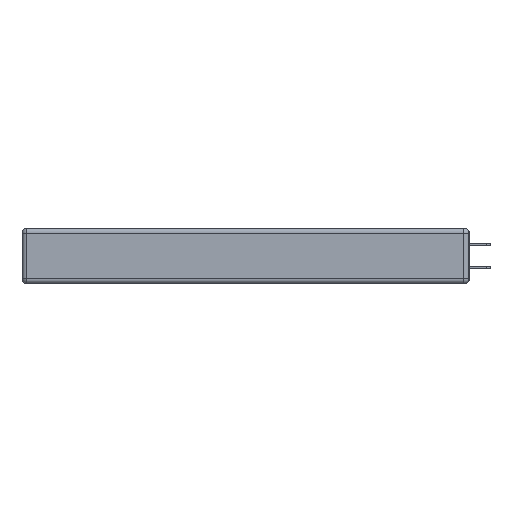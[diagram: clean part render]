
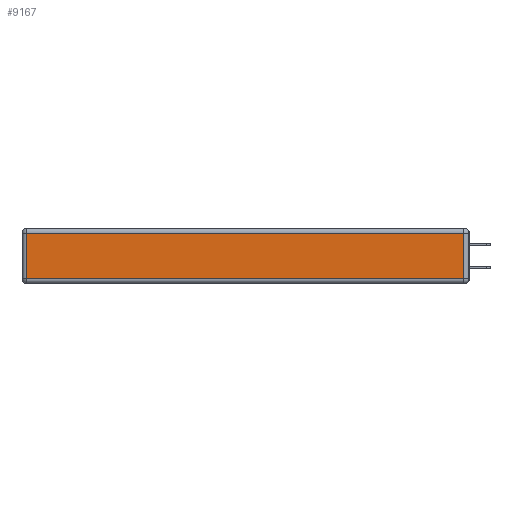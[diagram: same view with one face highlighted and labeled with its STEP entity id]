
A CAD part, left-side view. The second image highlights one B-rep face of the part: STEP entity #9167.
In plain terms, the highlighted planar face has unit normal (-1, 0, 0).
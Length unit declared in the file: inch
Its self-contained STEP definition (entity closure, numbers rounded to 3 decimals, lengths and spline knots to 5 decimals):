
#218 = PLANE ( 'NONE',  #24675 ) ;
#305 = DIRECTION ( 'NONE',  ( 0., 0., 1. ) ) ;
#1964 = VECTOR ( 'NONE', #5734, 39.37008 ) ;
#2726 = LINE ( 'NONE', #7223, #8931 ) ;
#2805 = CARTESIAN_POINT ( 'NONE',  ( 0., 0.03, -0.03 ) ) ;
#3046 = ORIENTED_EDGE ( 'NONE', *, *, #26388, .T. ) ;
#4100 = CARTESIAN_POINT ( 'NONE',  ( 0., 2.72, -0.343 ) ) ;
#4257 = LINE ( 'NONE', #4100, #1964 ) ;
#5115 = DIRECTION ( 'NONE',  ( 0., -1., 0. ) ) ;
#5734 = DIRECTION ( 'NONE',  ( 0., 0., -1. ) ) ;
#6194 = VERTEX_POINT ( 'NONE', #24801 ) ;
#7223 = CARTESIAN_POINT ( 'NONE',  ( 0., 0.03, -0.343 ) ) ;
#8496 = VECTOR ( 'NONE', #19951, 39.37008 ) ;
#8931 = VECTOR ( 'NONE', #13575, 39.37008 ) ;
#8938 = VERTEX_POINT ( 'NONE', #22077 ) ;
#9052 = CARTESIAN_POINT ( 'NONE',  ( 0., 0., -0.313 ) ) ;
#9167 = ADVANCED_FACE ( 'NONE', ( #10372 ), #218, .T. ) ;
#10372 = FACE_OUTER_BOUND ( 'NONE', #12320, .T. ) ;
#10502 = CARTESIAN_POINT ( 'NONE',  ( 0., 2.72, -0.313 ) ) ;
#11140 = VERTEX_POINT ( 'NONE', #10502 ) ;
#12320 = EDGE_LOOP ( 'NONE', ( #23861, #25351, #3046, #17737 ) ) ;
#12808 = DIRECTION ( 'NONE',  ( -1., 0., 0. ) ) ;
#13537 = VECTOR ( 'NONE', #5115, 39.37008 ) ;
#13575 = DIRECTION ( 'NONE',  ( 0., 0., 1. ) ) ;
#14387 = EDGE_CURVE ( 'NONE', #11140, #6194, #20064, .T. ) ;
#17737 = ORIENTED_EDGE ( 'NONE', *, *, #22283, .T. ) ;
#19107 = CARTESIAN_POINT ( 'NONE',  ( 0., 0., -0.343 ) ) ;
#19428 = VERTEX_POINT ( 'NONE', #2805 ) ;
#19571 = LINE ( 'NONE', #26121, #8496 ) ;
#19951 = DIRECTION ( 'NONE',  ( 0., 1., 0. ) ) ;
#20064 = LINE ( 'NONE', #9052, #13537 ) ;
#22077 = CARTESIAN_POINT ( 'NONE',  ( 0., 2.72, -0.03 ) ) ;
#22283 = EDGE_CURVE ( 'NONE', #8938, #11140, #4257, .T. ) ;
#23861 = ORIENTED_EDGE ( 'NONE', *, *, #14387, .T. ) ;
#24136 = EDGE_CURVE ( 'NONE', #6194, #19428, #2726, .T. ) ;
#24675 = AXIS2_PLACEMENT_3D ( 'NONE', #19107, #12808, #305 ) ;
#24801 = CARTESIAN_POINT ( 'NONE',  ( 0., 0.03, -0.313 ) ) ;
#25351 = ORIENTED_EDGE ( 'NONE', *, *, #24136, .T. ) ;
#26121 = CARTESIAN_POINT ( 'NONE',  ( 0., 2.75, -0.03 ) ) ;
#26388 = EDGE_CURVE ( 'NONE', #19428, #8938, #19571, .T. ) ;
